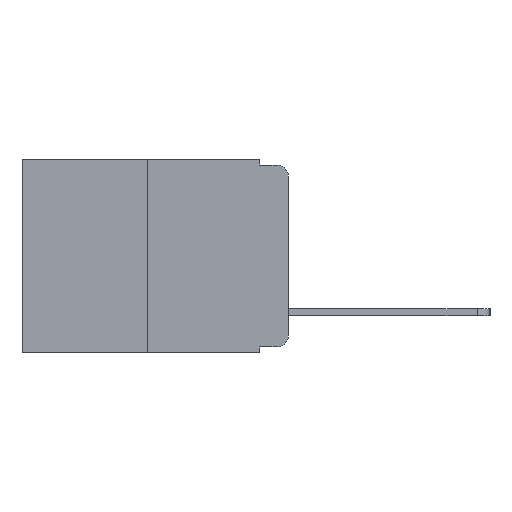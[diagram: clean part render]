
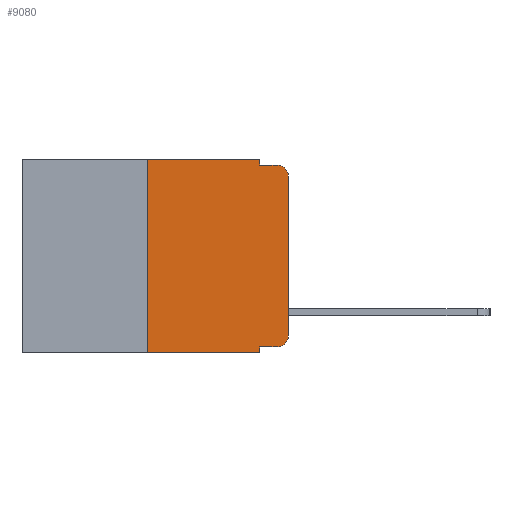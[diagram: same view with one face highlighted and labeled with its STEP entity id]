
A CAD part, left-side view. The second image highlights one B-rep face of the part: STEP entity #9080.
In plain terms, the highlighted planar face has unit normal (-1, 0, 0).
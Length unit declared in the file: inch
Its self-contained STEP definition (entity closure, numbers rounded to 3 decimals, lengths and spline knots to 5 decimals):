
#196 = ORIENTED_EDGE ( 'NONE', *, *, #1668, .F. ) ;
#516 = VERTEX_POINT ( 'NONE', #18418 ) ;
#614 = LINE ( 'NONE', #4845, #8452 ) ;
#690 = CARTESIAN_POINT ( 'NONE',  ( 0., 0., -0.313 ) ) ;
#937 = DIRECTION ( 'NONE',  ( -1., 0., 0. ) ) ;
#1283 = ORIENTED_EDGE ( 'NONE', *, *, #18846, .F. ) ;
#1668 = EDGE_CURVE ( 'NONE', #15745, #15779, #3684, .T. ) ;
#1809 = ORIENTED_EDGE ( 'NONE', *, *, #15515, .T. ) ;
#1947 = VERTEX_POINT ( 'NONE', #690 ) ;
#1951 = VERTEX_POINT ( 'NONE', #15755 ) ;
#1961 = DIRECTION ( 'NONE',  ( 0., -1., 0. ) ) ;
#2230 = VECTOR ( 'NONE', #1961, 39.37008 ) ;
#2768 = EDGE_CURVE ( 'NONE', #15779, #516, #21075, .T. ) ;
#2874 = CARTESIAN_POINT ( 'NONE',  ( 0., 0.473, -0.343 ) ) ;
#3207 = DIRECTION ( 'NONE',  ( 0., 0., 1. ) ) ;
#3684 = LINE ( 'NONE', #8058, #4216 ) ;
#3870 = EDGE_CURVE ( 'NONE', #16414, #516, #11998, .T. ) ;
#3906 = LINE ( 'NONE', #11588, #7826 ) ;
#4216 = VECTOR ( 'NONE', #6310, 39.37008 ) ;
#4507 = DIRECTION ( 'NONE',  ( 0., -1., 0. ) ) ;
#4611 = VECTOR ( 'NONE', #7192, 39.37008 ) ;
#4845 = CARTESIAN_POINT ( 'NONE',  ( 0., 0., 0. ) ) ;
#4848 = CARTESIAN_POINT ( 'NONE',  ( 0., 0.051, -0.01 ) ) ;
#4892 = CARTESIAN_POINT ( 'NONE',  ( 0., 0., -0.03 ) ) ;
#4967 = EDGE_CURVE ( 'NONE', #1947, #16414, #614, .T. ) ;
#5049 = PLANE ( 'NONE',  #15746 ) ;
#5114 = DIRECTION ( 'NONE',  ( 0., 0., -1. ) ) ;
#6289 = VERTEX_POINT ( 'NONE', #10509 ) ;
#6310 = DIRECTION ( 'NONE',  ( 0., 0., -1. ) ) ;
#7010 = CARTESIAN_POINT ( 'NONE',  ( 0., 0.25, -0.343 ) ) ;
#7092 = CARTESIAN_POINT ( 'NONE',  ( 0., 0.051, 0. ) ) ;
#7182 = LINE ( 'NONE', #16987, #2230 ) ;
#7192 = DIRECTION ( 'NONE',  ( 0., -1., 0. ) ) ;
#7534 = ORIENTED_EDGE ( 'NONE', *, *, #4967, .T. ) ;
#7765 = VECTOR ( 'NONE', #14569, 39.37008 ) ;
#7818 = VECTOR ( 'NONE', #4507, 39.37008 ) ;
#7826 = VECTOR ( 'NONE', #3207, 39.37008 ) ;
#8058 = CARTESIAN_POINT ( 'NONE',  ( 0., 0.051, 0. ) ) ;
#8452 = VECTOR ( 'NONE', #16586, 39.37008 ) ;
#9000 = LINE ( 'NONE', #7092, #17350 ) ;
#9080 = ADVANCED_FACE ( 'NONE', ( #17536 ), #5049, .F. ) ;
#9563 = DIRECTION ( 'NONE',  ( -1., 0., 0. ) ) ;
#9637 = LINE ( 'NONE', #10513, #4611 ) ;
#9650 = ORIENTED_EDGE ( 'NONE', *, *, #21018, .F. ) ;
#10509 = CARTESIAN_POINT ( 'NONE',  ( 0., 0.25, 0. ) ) ;
#10513 = CARTESIAN_POINT ( 'NONE',  ( 0., 0.051, -0.333 ) ) ;
#10649 = AXIS2_PLACEMENT_3D ( 'NONE', #19509, #9563, #21133 ) ;
#10751 = CARTESIAN_POINT ( 'NONE',  ( 0., 0.051, -0.343 ) ) ;
#10969 = CARTESIAN_POINT ( 'NONE',  ( 0., 0.02, -0.313 ) ) ;
#11512 = CARTESIAN_POINT ( 'NONE',  ( 0., 0.051, 0. ) ) ;
#11588 = CARTESIAN_POINT ( 'NONE',  ( 0., 0.25, 0. ) ) ;
#11722 = CARTESIAN_POINT ( 'NONE',  ( 0., 0.051, -0.333 ) ) ;
#11851 = CARTESIAN_POINT ( 'NONE',  ( 0., 0.473, 0. ) ) ;
#11998 = CIRCLE ( 'NONE', #10649, 0.02 ) ;
#12543 = ORIENTED_EDGE ( 'NONE', *, *, #3870, .T. ) ;
#12652 = DIRECTION ( 'NONE',  ( 0., 0., -1. ) ) ;
#13344 = EDGE_LOOP ( 'NONE', ( #7534, #12543, #16945, #196, #13577, #9650, #18503, #1283, #19017, #1809 ) ) ;
#13577 = ORIENTED_EDGE ( 'NONE', *, *, #18301, .F. ) ;
#13769 = VERTEX_POINT ( 'NONE', #10751 ) ;
#13969 = CIRCLE ( 'NONE', #19973, 0.02 ) ;
#14569 = DIRECTION ( 'NONE',  ( 0., -1., 0. ) ) ;
#15172 = DIRECTION ( 'NONE',  ( 1., 0., 0. ) ) ;
#15515 = EDGE_CURVE ( 'NONE', #1951, #1947, #13969, .T. ) ;
#15745 = VERTEX_POINT ( 'NONE', #11512 ) ;
#15746 = AXIS2_PLACEMENT_3D ( 'NONE', #11851, #15172, #5114 ) ;
#15755 = CARTESIAN_POINT ( 'NONE',  ( 0., 0.02, -0.333 ) ) ;
#15779 = VERTEX_POINT ( 'NONE', #4848 ) ;
#16099 = CARTESIAN_POINT ( 'NONE',  ( 0., 0.051, -0.01 ) ) ;
#16414 = VERTEX_POINT ( 'NONE', #4892 ) ;
#16586 = DIRECTION ( 'NONE',  ( 0., 0., 1. ) ) ;
#16627 = EDGE_CURVE ( 'NONE', #17699, #1951, #9637, .T. ) ;
#16667 = LINE ( 'NONE', #2874, #7765 ) ;
#16902 = EDGE_CURVE ( 'NONE', #20688, #13769, #16667, .T. ) ;
#16945 = ORIENTED_EDGE ( 'NONE', *, *, #2768, .F. ) ;
#16987 = CARTESIAN_POINT ( 'NONE',  ( 0., 0.473, 0. ) ) ;
#17350 = VECTOR ( 'NONE', #20403, 39.37008 ) ;
#17536 = FACE_OUTER_BOUND ( 'NONE', #13344, .T. ) ;
#17699 = VERTEX_POINT ( 'NONE', #11722 ) ;
#18301 = EDGE_CURVE ( 'NONE', #6289, #15745, #7182, .T. ) ;
#18418 = CARTESIAN_POINT ( 'NONE',  ( 0., 0.02, -0.01 ) ) ;
#18503 = ORIENTED_EDGE ( 'NONE', *, *, #16902, .T. ) ;
#18846 = EDGE_CURVE ( 'NONE', #17699, #13769, #9000, .T. ) ;
#19017 = ORIENTED_EDGE ( 'NONE', *, *, #16627, .T. ) ;
#19509 = CARTESIAN_POINT ( 'NONE',  ( 0., 0.02, -0.03 ) ) ;
#19973 = AXIS2_PLACEMENT_3D ( 'NONE', #10969, #937, #12652 ) ;
#20403 = DIRECTION ( 'NONE',  ( 0., 0., -1. ) ) ;
#20688 = VERTEX_POINT ( 'NONE', #7010 ) ;
#21018 = EDGE_CURVE ( 'NONE', #20688, #6289, #3906, .T. ) ;
#21075 = LINE ( 'NONE', #16099, #7818 ) ;
#21133 = DIRECTION ( 'NONE',  ( 0., 0., -1. ) ) ;
